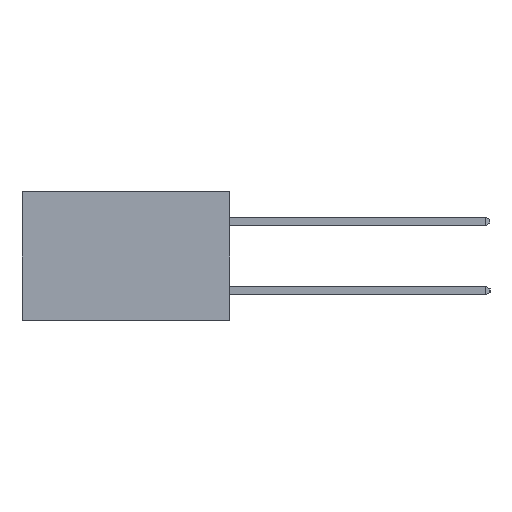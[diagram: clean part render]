
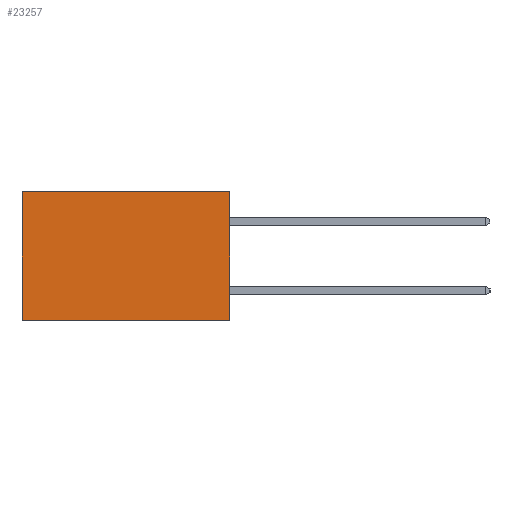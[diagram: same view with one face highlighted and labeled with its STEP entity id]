
A CAD part, left-side view. The second image highlights one B-rep face of the part: STEP entity #23257.
In plain terms, the highlighted planar face has unit normal (-1, 0, 0).
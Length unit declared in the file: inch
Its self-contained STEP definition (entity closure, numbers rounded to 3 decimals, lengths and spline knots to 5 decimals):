
#758 = CARTESIAN_POINT ( 'NONE',  ( 0.2615, 0., -0.37 ) ) ;
#1193 = EDGE_CURVE ( 'NONE', #16170, #15657, #12667, .T. ) ;
#2093 = LINE ( 'NONE', #758, #16898 ) ;
#4007 = DIRECTION ( 'NONE',  ( 0., 0., -1. ) ) ;
#4254 = AXIS2_PLACEMENT_3D ( 'NONE', #18397, #6492, #20358 ) ;
#5751 = ORIENTED_EDGE ( 'NONE', *, *, #24974, .F. ) ;
#6044 = CARTESIAN_POINT ( 'NONE',  ( 0.2615, 0.6, -0.37 ) ) ;
#6492 = DIRECTION ( 'NONE',  ( 1., 0., 0. ) ) ;
#7341 = VECTOR ( 'NONE', #4007, 39.37008 ) ;
#9198 = VECTOR ( 'NONE', #16549, 39.37008 ) ;
#9615 = VECTOR ( 'NONE', #13776, 39.37008 ) ;
#10351 = VERTEX_POINT ( 'NONE', #20344 ) ;
#11262 = CARTESIAN_POINT ( 'NONE',  ( 0.2615, 0., 0. ) ) ;
#11798 = CARTESIAN_POINT ( 'NONE',  ( 0.2615, 0., 0. ) ) ;
#12610 = CARTESIAN_POINT ( 'NONE',  ( 0.2615, 0., -0.37 ) ) ;
#12630 = VERTEX_POINT ( 'NONE', #11262 ) ;
#12667 = LINE ( 'NONE', #24445, #7341 ) ;
#13776 = DIRECTION ( 'NONE',  ( 0., 1., 0. ) ) ;
#14293 = ORIENTED_EDGE ( 'NONE', *, *, #1193, .T. ) ;
#14468 = LINE ( 'NONE', #12610, #9198 ) ;
#14568 = FACE_OUTER_BOUND ( 'NONE', #18568, .T. ) ;
#15657 = VERTEX_POINT ( 'NONE', #6044 ) ;
#16170 = VERTEX_POINT ( 'NONE', #17518 ) ;
#16549 = DIRECTION ( 'NONE',  ( 0., 0., -1. ) ) ;
#16661 = EDGE_CURVE ( 'NONE', #10351, #15657, #2093, .T. ) ;
#16898 = VECTOR ( 'NONE', #24634, 39.37008 ) ;
#17518 = CARTESIAN_POINT ( 'NONE',  ( 0.2615, 0.6, 0. ) ) ;
#18307 = PLANE ( 'NONE',  #4254 ) ;
#18397 = CARTESIAN_POINT ( 'NONE',  ( 0.2615, 0., -0.37 ) ) ;
#18568 = EDGE_LOOP ( 'NONE', ( #14293, #20139, #5751, #20233 ) ) ;
#19891 = EDGE_CURVE ( 'NONE', #12630, #16170, #24636, .T. ) ;
#20139 = ORIENTED_EDGE ( 'NONE', *, *, #16661, .F. ) ;
#20233 = ORIENTED_EDGE ( 'NONE', *, *, #19891, .T. ) ;
#20344 = CARTESIAN_POINT ( 'NONE',  ( 0.2615, 0., -0.37 ) ) ;
#20358 = DIRECTION ( 'NONE',  ( 0., 0., -1. ) ) ;
#23257 = ADVANCED_FACE ( 'NONE', ( #14568 ), #18307, .F. ) ;
#24445 = CARTESIAN_POINT ( 'NONE',  ( 0.2615, 0.6, -0.37 ) ) ;
#24634 = DIRECTION ( 'NONE',  ( 0., 1., 0. ) ) ;
#24636 = LINE ( 'NONE', #11798, #9615 ) ;
#24974 = EDGE_CURVE ( 'NONE', #12630, #10351, #14468, .T. ) ;
